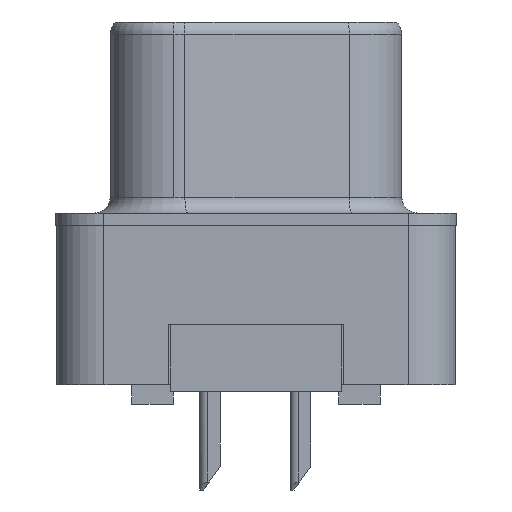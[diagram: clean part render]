
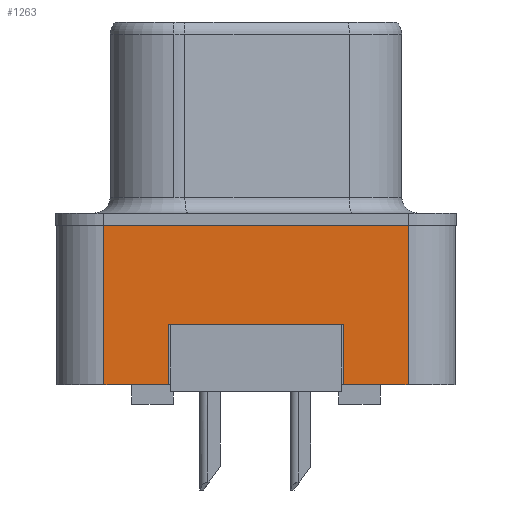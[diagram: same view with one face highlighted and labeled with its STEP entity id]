
A CAD part, left-side view. The second image highlights one B-rep face of the part: STEP entity #1263.
In plain terms, the highlighted planar face has unit normal (-1, 0, 0).
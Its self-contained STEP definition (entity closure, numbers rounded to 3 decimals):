
#160 = VERTEX_POINT ( 'NONE', #10717 ) ;
#436 = VECTOR ( 'NONE', #5245, 1000. ) ;
#581 = CARTESIAN_POINT ( 'NONE',  ( -2.935, 2.75, -3.1 ) ) ;
#856 = VERTEX_POINT ( 'NONE', #10470 ) ;
#879 = VERTEX_POINT ( 'NONE', #6177 ) ;
#1175 = CARTESIAN_POINT ( 'NONE',  ( -2.935, -2.75, -3.1 ) ) ;
#1223 = CARTESIAN_POINT ( 'NONE',  ( -2.935, -2.75, -3.1 ) ) ;
#1263 = ADVANCED_FACE ( 'NONE', ( #5867 ), #13232, .T. ) ;
#1555 = ORIENTED_EDGE ( 'NONE', *, *, #6730, .F. ) ;
#2607 = CARTESIAN_POINT ( 'NONE',  ( -2.935, -4.775, -5. ) ) ;
#3183 = CARTESIAN_POINT ( 'NONE',  ( -2.935, -4.775, -5. ) ) ;
#3418 = LINE ( 'NONE', #16424, #16339 ) ;
#4035 = LINE ( 'NONE', #1175, #4703 ) ;
#4412 = DIRECTION ( 'NONE',  ( 0., 0., -1. ) ) ;
#4490 = EDGE_CURVE ( 'NONE', #12151, #14433, #13861, .T. ) ;
#4527 = DIRECTION ( 'NONE',  ( -1., 0., 0. ) ) ;
#4703 = VECTOR ( 'NONE', #4412, 1000. ) ;
#5245 = DIRECTION ( 'NONE',  ( 0., 0., -1. ) ) ;
#5542 = EDGE_CURVE ( 'NONE', #879, #14433, #16687, .T. ) ;
#5867 = FACE_OUTER_BOUND ( 'NONE', #7189, .T. ) ;
#5955 = CARTESIAN_POINT ( 'NONE',  ( -2.935, -4.775, -5. ) ) ;
#6118 = CARTESIAN_POINT ( 'NONE',  ( -2.935, -4.775, -5. ) ) ;
#6177 = CARTESIAN_POINT ( 'NONE',  ( -2.935, 4.775, 0. ) ) ;
#6241 = DIRECTION ( 'NONE',  ( 0., -1., 0. ) ) ;
#6500 = LINE ( 'NONE', #6684, #436 ) ;
#6636 = VECTOR ( 'NONE', #6241, 1000. ) ;
#6684 = CARTESIAN_POINT ( 'NONE',  ( -2.935, 2.75, -3.1 ) ) ;
#6730 = EDGE_CURVE ( 'NONE', #7002, #16049, #12241, .T. ) ;
#6823 = CARTESIAN_POINT ( 'NONE',  ( -2.935, -4.775, 0. ) ) ;
#7002 = VERTEX_POINT ( 'NONE', #1223 ) ;
#7189 = EDGE_LOOP ( 'NONE', ( #8611, #17267, #17333, #10842, #12510, #17576, #14957, #1555 ) ) ;
#7927 = CARTESIAN_POINT ( 'NONE',  ( -2.935, 2.75, -3.1 ) ) ;
#8430 = VECTOR ( 'NONE', #18526, 1000. ) ;
#8611 = ORIENTED_EDGE ( 'NONE', *, *, #9275, .T. ) ;
#8924 = DIRECTION ( 'NONE',  ( 0., 0., 1. ) ) ;
#9275 = EDGE_CURVE ( 'NONE', #7002, #160, #4035, .T. ) ;
#10470 = CARTESIAN_POINT ( 'NONE',  ( -2.935, 4.775, -5. ) ) ;
#10717 = CARTESIAN_POINT ( 'NONE',  ( -2.935, -2.75, -5. ) ) ;
#10820 = LINE ( 'NONE', #3183, #6636 ) ;
#10842 = ORIENTED_EDGE ( 'NONE', *, *, #5542, .F. ) ;
#11145 = DIRECTION ( 'NONE',  ( 0., -1., 0. ) ) ;
#11194 = EDGE_CURVE ( 'NONE', #16049, #17682, #6500, .T. ) ;
#11510 = EDGE_CURVE ( 'NONE', #856, #879, #3418, .T. ) ;
#11700 = CARTESIAN_POINT ( 'NONE',  ( -2.935, 2.75, -5. ) ) ;
#12034 = DIRECTION ( 'NONE',  ( 0., 1., 0. ) ) ;
#12151 = VERTEX_POINT ( 'NONE', #2607 ) ;
#12241 = LINE ( 'NONE', #7927, #14625 ) ;
#12510 = ORIENTED_EDGE ( 'NONE', *, *, #11510, .F. ) ;
#13232 = PLANE ( 'NONE',  #14758 ) ;
#13819 = DIRECTION ( 'NONE',  ( 0., -1., 0. ) ) ;
#13861 = LINE ( 'NONE', #6118, #8430 ) ;
#13995 = VECTOR ( 'NONE', #11145, 1000. ) ;
#14271 = EDGE_CURVE ( 'NONE', #160, #12151, #10820, .T. ) ;
#14433 = VERTEX_POINT ( 'NONE', #18562 ) ;
#14579 = VECTOR ( 'NONE', #13819, 1000. ) ;
#14625 = VECTOR ( 'NONE', #12034, 1000. ) ;
#14758 = AXIS2_PLACEMENT_3D ( 'NONE', #5955, #4527, #8924 ) ;
#14957 = ORIENTED_EDGE ( 'NONE', *, *, #11194, .F. ) ;
#14998 = DIRECTION ( 'NONE',  ( 0., 0., 1. ) ) ;
#15100 = LINE ( 'NONE', #16905, #13995 ) ;
#15302 = EDGE_CURVE ( 'NONE', #856, #17682, #15100, .T. ) ;
#16049 = VERTEX_POINT ( 'NONE', #581 ) ;
#16339 = VECTOR ( 'NONE', #14998, 1000. ) ;
#16424 = CARTESIAN_POINT ( 'NONE',  ( -2.935, 4.775, -5. ) ) ;
#16687 = LINE ( 'NONE', #6823, #14579 ) ;
#16905 = CARTESIAN_POINT ( 'NONE',  ( -2.935, -4.775, -5. ) ) ;
#17267 = ORIENTED_EDGE ( 'NONE', *, *, #14271, .T. ) ;
#17333 = ORIENTED_EDGE ( 'NONE', *, *, #4490, .T. ) ;
#17576 = ORIENTED_EDGE ( 'NONE', *, *, #15302, .T. ) ;
#17682 = VERTEX_POINT ( 'NONE', #11700 ) ;
#18526 = DIRECTION ( 'NONE',  ( 0., 0., 1. ) ) ;
#18562 = CARTESIAN_POINT ( 'NONE',  ( -2.935, -4.775, 0. ) ) ;
